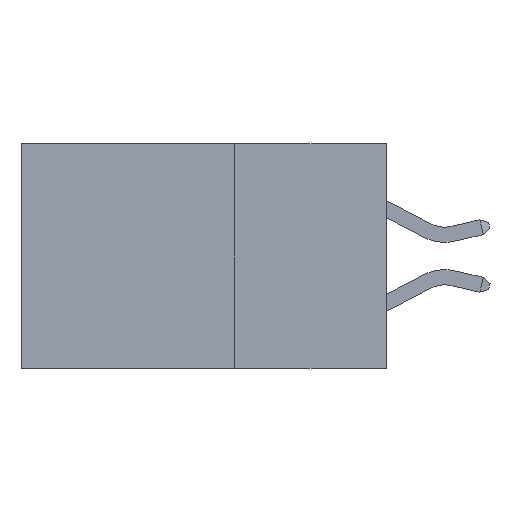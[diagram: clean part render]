
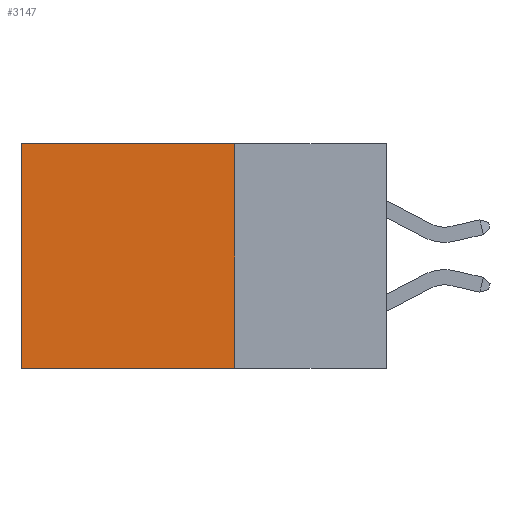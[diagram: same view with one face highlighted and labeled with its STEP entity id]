
A CAD part, left-side view. The second image highlights one B-rep face of the part: STEP entity #3147.
In plain terms, the highlighted planar face has unit normal (-1, 0, 0).
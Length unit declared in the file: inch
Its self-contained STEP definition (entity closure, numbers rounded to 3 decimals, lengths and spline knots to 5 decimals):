
#125 = CARTESIAN_POINT ( 'NONE',  ( 0.2615, 0.25, 0. ) ) ;
#863 = VECTOR ( 'NONE', #16033, 39.37008 ) ;
#1299 = EDGE_CURVE ( 'NONE', #2887, #9744, #10509, .T. ) ;
#1327 = VERTEX_POINT ( 'NONE', #2970 ) ;
#2887 = VERTEX_POINT ( 'NONE', #5013 ) ;
#2970 = CARTESIAN_POINT ( 'NONE',  ( 0.2615, 0.6, -0.37 ) ) ;
#3054 = AXIS2_PLACEMENT_3D ( 'NONE', #23715, #23550, #23549 ) ;
#3116 = FACE_OUTER_BOUND ( 'NONE', #16841, .T. ) ;
#3147 = ADVANCED_FACE ( 'NONE', ( #3116 ), #23601, .F. ) ;
#3823 = ORIENTED_EDGE ( 'NONE', *, *, #9080, .F. ) ;
#4130 = CARTESIAN_POINT ( 'NONE',  ( 0.2615, 0.25, -0.37 ) ) ;
#4156 = DIRECTION ( 'NONE',  ( 0., 1., 0. ) ) ;
#4253 = CARTESIAN_POINT ( 'NONE',  ( 0.2615, 0.6, -0.37 ) ) ;
#5013 = CARTESIAN_POINT ( 'NONE',  ( 0.2615, 0.25, 0. ) ) ;
#6065 = DIRECTION ( 'NONE',  ( 0., 0., -1. ) ) ;
#8057 = ORIENTED_EDGE ( 'NONE', *, *, #24410, .T. ) ;
#8985 = CARTESIAN_POINT ( 'NONE',  ( 0.2615, 0.25, -0.37 ) ) ;
#9080 = EDGE_CURVE ( 'NONE', #9744, #1327, #22345, .T. ) ;
#9744 = VERTEX_POINT ( 'NONE', #4130 ) ;
#10509 = LINE ( 'NONE', #8985, #20195 ) ;
#11421 = LINE ( 'NONE', #4253, #863 ) ;
#12856 = VERTEX_POINT ( 'NONE', #19143 ) ;
#13698 = EDGE_CURVE ( 'NONE', #12856, #1327, #11421, .T. ) ;
#14439 = DIRECTION ( 'NONE',  ( 0., 1., 0. ) ) ;
#14781 = CARTESIAN_POINT ( 'NONE',  ( 0.2615, 0.25, -0.37 ) ) ;
#16033 = DIRECTION ( 'NONE',  ( 0., 0., -1. ) ) ;
#16841 = EDGE_LOOP ( 'NONE', ( #19695, #3823, #23869, #8057 ) ) ;
#17269 = VECTOR ( 'NONE', #14439, 39.37008 ) ;
#17765 = VECTOR ( 'NONE', #4156, 39.37008 ) ;
#19143 = CARTESIAN_POINT ( 'NONE',  ( 0.2615, 0.6, 0. ) ) ;
#19695 = ORIENTED_EDGE ( 'NONE', *, *, #13698, .T. ) ;
#20195 = VECTOR ( 'NONE', #6065, 39.37008 ) ;
#22345 = LINE ( 'NONE', #14781, #17269 ) ;
#22843 = LINE ( 'NONE', #125, #17765 ) ;
#23549 = DIRECTION ( 'NONE',  ( 0., 0., -1. ) ) ;
#23550 = DIRECTION ( 'NONE',  ( 1., 0., 0. ) ) ;
#23601 = PLANE ( 'NONE',  #3054 ) ;
#23715 = CARTESIAN_POINT ( 'NONE',  ( 0.2615, 0.25, -0.37 ) ) ;
#23869 = ORIENTED_EDGE ( 'NONE', *, *, #1299, .F. ) ;
#24410 = EDGE_CURVE ( 'NONE', #2887, #12856, #22843, .T. ) ;
